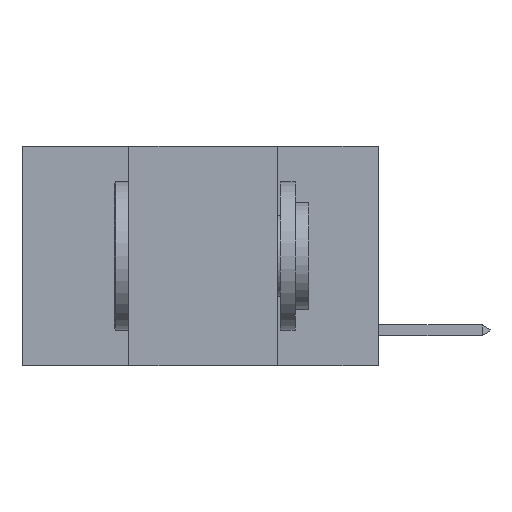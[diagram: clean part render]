
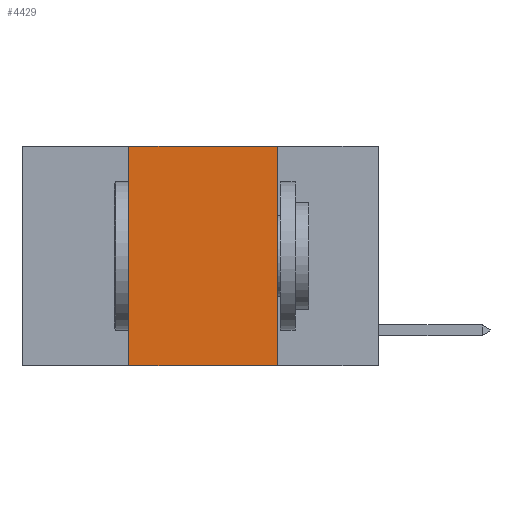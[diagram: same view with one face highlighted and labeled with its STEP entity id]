
A CAD part, left-side view. The second image highlights one B-rep face of the part: STEP entity #4429.
In plain terms, the highlighted planar face has unit normal (-1, 0, 0).
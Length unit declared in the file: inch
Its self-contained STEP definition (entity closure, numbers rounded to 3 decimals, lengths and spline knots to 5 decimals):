
#327 = ORIENTED_EDGE ( 'NONE', *, *, #21991, .T. ) ;
#761 = VERTEX_POINT ( 'NONE', #18504 ) ;
#1682 = CARTESIAN_POINT ( 'NONE',  ( 0., 0.42, 0. ) ) ;
#1737 = VECTOR ( 'NONE', #3608, 39.37008 ) ;
#2740 = ORIENTED_EDGE ( 'NONE', *, *, #9222, .F. ) ;
#3099 = VECTOR ( 'NONE', #19020, 39.37008 ) ;
#3608 = DIRECTION ( 'NONE',  ( 0., 0., 1. ) ) ;
#3749 = DIRECTION ( 'NONE',  ( 0., 0., -1. ) ) ;
#3867 = VERTEX_POINT ( 'NONE', #17702 ) ;
#4201 = EDGE_LOOP ( 'NONE', ( #2740, #18877, #19457, #327 ) ) ;
#4255 = LINE ( 'NONE', #5172, #22405 ) ;
#4429 = ADVANCED_FACE ( 'NONE', ( #20675 ), #13420, .F. ) ;
#5172 = CARTESIAN_POINT ( 'NONE',  ( 0., 0.6, 0. ) ) ;
#5902 = CARTESIAN_POINT ( 'NONE',  ( 0., 0.17, 0. ) ) ;
#6915 = LINE ( 'NONE', #1682, #1737 ) ;
#7130 = DIRECTION ( 'NONE',  ( 0., -1., 0. ) ) ;
#9222 = EDGE_CURVE ( 'NONE', #14429, #12653, #21017, .T. ) ;
#10732 = VECTOR ( 'NONE', #13118, 39.37008 ) ;
#11070 = AXIS2_PLACEMENT_3D ( 'NONE', #21121, #15357, #3749 ) ;
#11095 = EDGE_CURVE ( 'NONE', #761, #14429, #4255, .T. ) ;
#11182 = CARTESIAN_POINT ( 'NONE',  ( 0., 0.17, 0. ) ) ;
#12653 = VERTEX_POINT ( 'NONE', #17608 ) ;
#13118 = DIRECTION ( 'NONE',  ( 0., 0., -1. ) ) ;
#13420 = PLANE ( 'NONE',  #11070 ) ;
#14429 = VERTEX_POINT ( 'NONE', #5902 ) ;
#15357 = DIRECTION ( 'NONE',  ( 1., 0., 0. ) ) ;
#17608 = CARTESIAN_POINT ( 'NONE',  ( 0., 0.17, -0.37 ) ) ;
#17702 = CARTESIAN_POINT ( 'NONE',  ( 0., 0.42, -0.37 ) ) ;
#18504 = CARTESIAN_POINT ( 'NONE',  ( 0., 0.42, 0. ) ) ;
#18610 = LINE ( 'NONE', #24707, #3099 ) ;
#18877 = ORIENTED_EDGE ( 'NONE', *, *, #11095, .F. ) ;
#19020 = DIRECTION ( 'NONE',  ( 0., -1., 0. ) ) ;
#19457 = ORIENTED_EDGE ( 'NONE', *, *, #19593, .F. ) ;
#19593 = EDGE_CURVE ( 'NONE', #3867, #761, #6915, .T. ) ;
#20675 = FACE_OUTER_BOUND ( 'NONE', #4201, .T. ) ;
#21017 = LINE ( 'NONE', #11182, #10732 ) ;
#21121 = CARTESIAN_POINT ( 'NONE',  ( 0., 0.6, 0. ) ) ;
#21991 = EDGE_CURVE ( 'NONE', #3867, #12653, #18610, .T. ) ;
#22405 = VECTOR ( 'NONE', #7130, 39.37008 ) ;
#24707 = CARTESIAN_POINT ( 'NONE',  ( 0., 0.6, -0.37 ) ) ;
